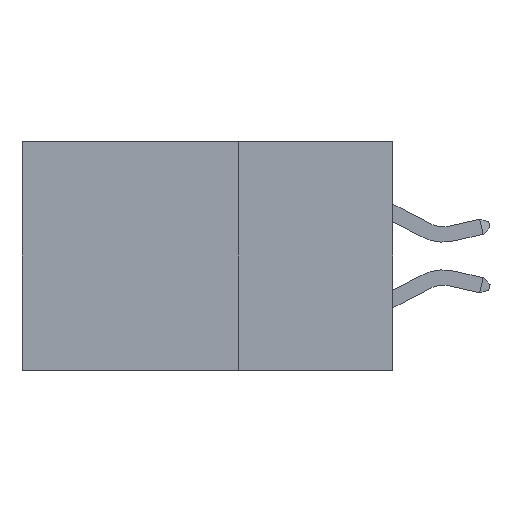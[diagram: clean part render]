
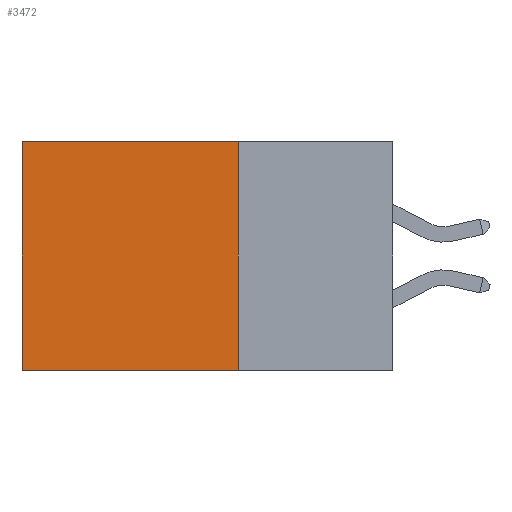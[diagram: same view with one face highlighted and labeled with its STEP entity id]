
A CAD part, left-side view. The second image highlights one B-rep face of the part: STEP entity #3472.
In plain terms, the highlighted planar face has unit normal (-1, 0, 0).
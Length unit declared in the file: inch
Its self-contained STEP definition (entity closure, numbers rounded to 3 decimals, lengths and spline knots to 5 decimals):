
#55 = VECTOR ( 'NONE', #10929, 39.37008 ) ;
#1088 = ORIENTED_EDGE ( 'NONE', *, *, #7358, .T. ) ;
#2454 = VECTOR ( 'NONE', #3100, 39.37008 ) ;
#2505 = ORIENTED_EDGE ( 'NONE', *, *, #2542, .F. ) ;
#2542 = EDGE_CURVE ( 'NONE', #9666, #2774, #2803, .T. ) ;
#2774 = VERTEX_POINT ( 'NONE', #9246 ) ;
#2803 = LINE ( 'NONE', #4171, #8157 ) ;
#3003 = CARTESIAN_POINT ( 'NONE',  ( 0.2875, 0.6, 0. ) ) ;
#3100 = DIRECTION ( 'NONE',  ( 0., 0., -1. ) ) ;
#3215 = CARTESIAN_POINT ( 'NONE',  ( 0.2875, 0.25, 0. ) ) ;
#3472 = ADVANCED_FACE ( 'NONE', ( #5351 ), #9235, .F. ) ;
#4021 = DIRECTION ( 'NONE',  ( 0., 0., -1. ) ) ;
#4089 = CARTESIAN_POINT ( 'NONE',  ( 0.2875, 0.25, 0. ) ) ;
#4099 = VERTEX_POINT ( 'NONE', #6696 ) ;
#4171 = CARTESIAN_POINT ( 'NONE',  ( 0.2875, 0.25, -0.37 ) ) ;
#4734 = CARTESIAN_POINT ( 'NONE',  ( 0.2875, 0.25, 0. ) ) ;
#4816 = AXIS2_PLACEMENT_3D ( 'NONE', #3215, #6704, #4021 ) ;
#4994 = DIRECTION ( 'NONE',  ( 0., 1., 0. ) ) ;
#5351 = FACE_OUTER_BOUND ( 'NONE', #10980, .T. ) ;
#5827 = LINE ( 'NONE', #3003, #2454 ) ;
#5885 = DIRECTION ( 'NONE',  ( 0., 1., 0. ) ) ;
#5984 = VECTOR ( 'NONE', #4994, 39.37008 ) ;
#6696 = CARTESIAN_POINT ( 'NONE',  ( 0.2875, 0.25, 0. ) ) ;
#6704 = DIRECTION ( 'NONE',  ( 1., 0., 0. ) ) ;
#6880 = ORIENTED_EDGE ( 'NONE', *, *, #8620, .F. ) ;
#6991 = ORIENTED_EDGE ( 'NONE', *, *, #8496, .T. ) ;
#7358 = EDGE_CURVE ( 'NONE', #4099, #8650, #10802, .T. ) ;
#8037 = CARTESIAN_POINT ( 'NONE',  ( 0.2875, 0.25, -0.37 ) ) ;
#8157 = VECTOR ( 'NONE', #5885, 39.37008 ) ;
#8496 = EDGE_CURVE ( 'NONE', #8650, #2774, #5827, .T. ) ;
#8620 = EDGE_CURVE ( 'NONE', #4099, #9666, #9283, .T. ) ;
#8650 = VERTEX_POINT ( 'NONE', #9187 ) ;
#9187 = CARTESIAN_POINT ( 'NONE',  ( 0.2875, 0.6, 0. ) ) ;
#9235 = PLANE ( 'NONE',  #4816 ) ;
#9246 = CARTESIAN_POINT ( 'NONE',  ( 0.2875, 0.6, -0.37 ) ) ;
#9283 = LINE ( 'NONE', #4734, #55 ) ;
#9666 = VERTEX_POINT ( 'NONE', #8037 ) ;
#10802 = LINE ( 'NONE', #4089, #5984 ) ;
#10929 = DIRECTION ( 'NONE',  ( 0., 0., -1. ) ) ;
#10980 = EDGE_LOOP ( 'NONE', ( #6991, #2505, #6880, #1088 ) ) ;
